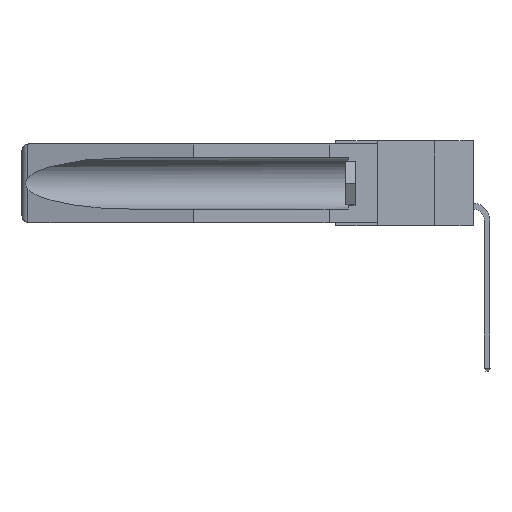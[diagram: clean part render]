
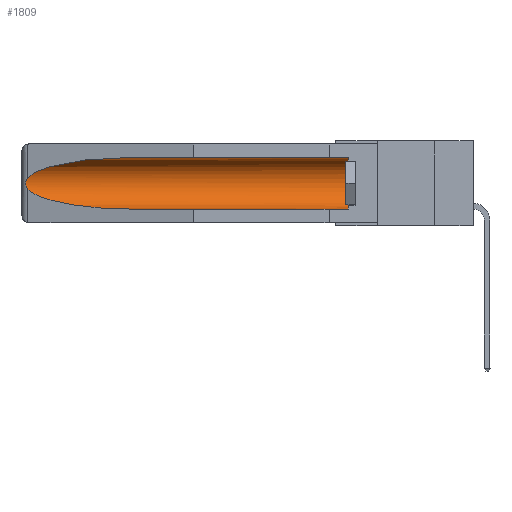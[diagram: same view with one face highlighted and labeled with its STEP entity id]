
A CAD part, left-side view. The second image highlights one B-rep face of the part: STEP entity #1809.
In plain terms, the highlighted cylindrical face has radius 2.857 mm (diameter 5.715 mm), a partial arc.
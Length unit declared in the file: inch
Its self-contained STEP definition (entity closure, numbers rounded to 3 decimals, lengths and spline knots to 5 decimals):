
#513 = CARTESIAN_POINT ( 'NONE',  ( 0.26597, 1.52961, -0.15275 ) ) ;
#593 = CARTESIAN_POINT ( 'NONE',  ( 0.26537, 1.52718, -0.19328 ) ) ;
#1071 = CARTESIAN_POINT ( 'NONE',  ( 0.21114, 1.30732, -0.284 ) ) ;
#1679 = CARTESIAN_POINT ( 'NONE',  ( 0.155, 1.07973, -0.059 ) ) ;
#1809 = ADVANCED_FACE ( 'NONE', ( #20720 ), #24072, .F. ) ;
#1831 = VECTOR ( 'NONE', #15468, 39.37008 ) ;
#2150 = LINE ( 'NONE', #22961, #1831 ) ;
#3261 = DIRECTION ( 'NONE',  ( 0., 1., 0. ) ) ;
#3644 = VERTEX_POINT ( 'NONE', #5999 ) ;
#3726 = EDGE_CURVE ( 'NONE', #11166, #5113, #19826, .T. ) ;
#4094 = ORIENTED_EDGE ( 'NONE', *, *, #3726, .T. ) ;
#4436 = CARTESIAN_POINT ( 'NONE',  ( 0.2673, 1.5327, -0.16383 ) ) ;
#5113 = VERTEX_POINT ( 'NONE', #11446 ) ;
#5492 = CARTESIAN_POINT ( 'NONE',  ( 0.155, -0.30754, -0.059 ) ) ;
#5950 = ORIENTED_EDGE ( 'NONE', *, *, #24000, .T. ) ;
#5999 = CARTESIAN_POINT ( 'NONE',  ( 0.155, 1.07973, -0.284 ) ) ;
#6300 = EDGE_CURVE ( 'NONE', #17392, #3644, #2150, .T. ) ;
#6870 = ORIENTED_EDGE ( 'NONE', *, *, #19281, .T. ) ;
#7668 = ORIENTED_EDGE ( 'NONE', *, *, #6300, .F. ) ;
#7786 = CARTESIAN_POINT ( 'NONE',  ( 0.26537, 1.52718, -0.14972 ) ) ;
#8213 = AXIS2_PLACEMENT_3D ( 'NONE', #8390, #21825, #14147 ) ;
#8358 = CARTESIAN_POINT ( 'NONE',  ( 0.2675, 1.53308, -0.17534 ) ) ;
#8390 = CARTESIAN_POINT ( 'NONE',  ( 0.155, 0.126, -0.1715 ) ) ;
#8765 = CARTESIAN_POINT ( 'NONE',  ( 0.155, 1.07973, -0.284 ) ) ;
#8887 = LINE ( 'NONE', #5492, #11643 ) ;
#9620 = CIRCLE ( 'NONE', #8213, 0.1125 ) ;
#9720 = CARTESIAN_POINT ( 'NONE',  ( 0.25451, 1.48313, -0.09465 ) ) ;
#9828 = ORIENTED_EDGE ( 'NONE', *, *, #13418, .T. ) ;
#10565 = CARTESIAN_POINT ( 'NONE',  ( 0.26537, 1.52718, -0.19328 ) ) ;
#11166 = VERTEX_POINT ( 'NONE', #7786 ) ;
#11446 = CARTESIAN_POINT ( 'NONE',  ( 0.26537, 1.52718, -0.19328 ) ) ;
#11643 = VECTOR ( 'NONE', #19174, 39.37008 ) ;
#12811 = DIRECTION ( 'NONE',  ( 0., 0., 1. ) ) ;
#13418 = EDGE_CURVE ( 'NONE', #22262, #11166, #18237, .T. ) ;
#14147 = DIRECTION ( 'NONE',  ( 0., 0., 1. ) ) ;
#14206 = CARTESIAN_POINT ( 'NONE',  ( 0.26654, 1.53092, -0.15636 ) ) ;
#15384 = EDGE_LOOP ( 'NONE', ( #9828, #4094, #5950, #7668, #17705, #6870 ) ) ;
#15468 = DIRECTION ( 'NONE',  ( 0., 1., 0. ) ) ;
#15752 = CARTESIAN_POINT ( 'NONE',  ( 0.155, 0.126, -0.284 ) ) ;
#15784 = CARTESIAN_POINT ( 'NONE',  ( 0.26537, 1.52718, -0.14972 ) ) ;
#16083 = CARTESIAN_POINT ( 'NONE',  ( 0.26537, 1.52718, -0.14972 ) ) ;
#16594 = VERTEX_POINT ( 'NONE', #21949 ) ;
#16937 = AXIS2_PLACEMENT_3D ( 'NONE', #24261, #3261, #12811 ) ;
#17392 = VERTEX_POINT ( 'NONE', #15752 ) ;
#17705 = ORIENTED_EDGE ( 'NONE', *, *, #25278, .T. ) ;
#17934 = CARTESIAN_POINT ( 'NONE',  ( 0.26597, 1.5296, -0.19026 ) ) ;
#18237 =( BOUNDED_CURVE ( )  B_SPLINE_CURVE ( 3, ( #1679, #25243, #9720, #15784 ),
 .UNSPECIFIED., .F., .F. ) 
 B_SPLINE_CURVE_WITH_KNOTS ( ( 4, 4 ),
 ( 4.71239, 6.08839 ),
 .UNSPECIFIED. ) 
 CURVE ( )  GEOMETRIC_REPRESENTATION_ITEM ( )  RATIONAL_B_SPLINE_CURVE ( ( 1., 0.848, 0.848, 1. ) ) 
 REPRESENTATION_ITEM ( '' )  );
#18411 = CARTESIAN_POINT ( 'NONE',  ( 0.25451, 1.48313, -0.24835 ) ) ;
#18476 = CARTESIAN_POINT ( 'NONE',  ( 0.155, 1.07973, -0.059 ) ) ;
#19174 = DIRECTION ( 'NONE',  ( 0., 1., 0. ) ) ;
#19281 = EDGE_CURVE ( 'NONE', #16594, #22262, #8887, .T. ) ;
#19826 = B_SPLINE_CURVE_WITH_KNOTS ( 'NONE', 3,
 ( #16083, #513, #14206, #4436, #23742, #8358, #22032, #23990, #17934, #593 ),
 .UNSPECIFIED., .F., .F.,
 ( 4, 2, 2, 2, 4 ),
 ( 0., 0.00029, 0.00058, 0.00087, 0.00117 ),
 .UNSPECIFIED. ) ;
#20720 = FACE_OUTER_BOUND ( 'NONE', #15384, .T. ) ;
#21825 = DIRECTION ( 'NONE',  ( 0., -1., 0. ) ) ;
#21949 = CARTESIAN_POINT ( 'NONE',  ( 0.155, 0.126, -0.059 ) ) ;
#22032 = CARTESIAN_POINT ( 'NONE',  ( 0.2673, 1.53269, -0.17917 ) ) ;
#22262 = VERTEX_POINT ( 'NONE', #18476 ) ;
#22961 = CARTESIAN_POINT ( 'NONE',  ( 0.155, -0.30754, -0.284 ) ) ;
#23581 =( BOUNDED_CURVE ( )  B_SPLINE_CURVE ( 3, ( #10565, #18411, #1071, #8765 ),
 .UNSPECIFIED., .F., .F. ) 
 B_SPLINE_CURVE_WITH_KNOTS ( ( 4, 4 ),
 ( 0.1948, 1.5708 ),
 .UNSPECIFIED. ) 
 CURVE ( )  GEOMETRIC_REPRESENTATION_ITEM ( )  RATIONAL_B_SPLINE_CURVE ( ( 1., 0.848, 0.848, 1. ) ) 
 REPRESENTATION_ITEM ( '' )  );
#23742 = CARTESIAN_POINT ( 'NONE',  ( 0.2675, 1.53308, -0.16763 ) ) ;
#23990 = CARTESIAN_POINT ( 'NONE',  ( 0.26655, 1.53094, -0.18657 ) ) ;
#24000 = EDGE_CURVE ( 'NONE', #5113, #3644, #23581, .T. ) ;
#24072 = CYLINDRICAL_SURFACE ( 'NONE', #16937, 0.1125 ) ;
#24261 = CARTESIAN_POINT ( 'NONE',  ( 0.155, -0.30754, -0.1715 ) ) ;
#25243 = CARTESIAN_POINT ( 'NONE',  ( 0.21114, 1.30732, -0.059 ) ) ;
#25278 = EDGE_CURVE ( 'NONE', #17392, #16594, #9620, .T. ) ;
